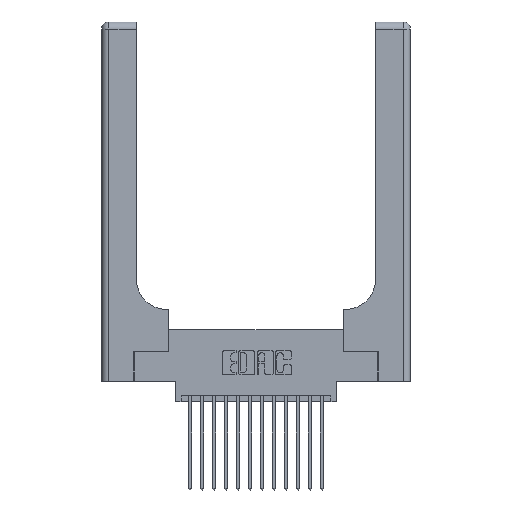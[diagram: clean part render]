
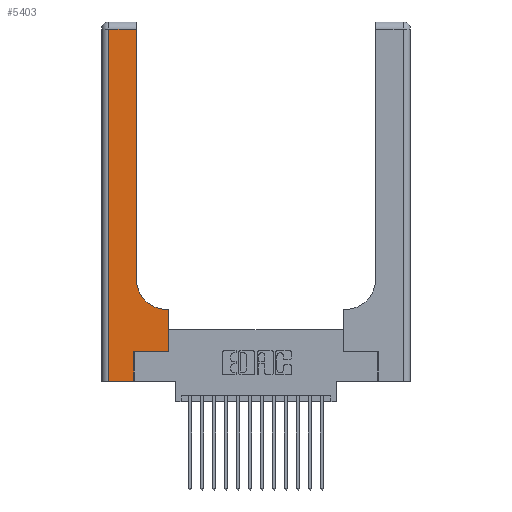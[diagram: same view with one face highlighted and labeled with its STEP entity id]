
A CAD part, top view. The second image highlights one B-rep face of the part: STEP entity #5403.
In plain terms, the highlighted planar face has unit normal (0, 0, 1).
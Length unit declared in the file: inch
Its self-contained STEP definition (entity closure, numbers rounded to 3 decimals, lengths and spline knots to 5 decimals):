
#266 = CARTESIAN_POINT ( 'NONE',  ( 0.269, 0.25, 0.37 ) ) ;
#598 = DIRECTION ( 'NONE',  ( -1., 0., 0. ) ) ;
#629 = CARTESIAN_POINT ( 'NONE',  ( 0.5585, 0.6, 0.37 ) ) ;
#652 = VECTOR ( 'NONE', #2944, 39.37008 ) ;
#919 = EDGE_CURVE ( 'NONE', #15310, #13263, #16381, .T. ) ;
#1130 = DIRECTION ( 'NONE',  ( 0., 1., 0. ) ) ;
#1141 = LINE ( 'NONE', #266, #12323 ) ;
#1341 = ORIENTED_EDGE ( 'NONE', *, *, #3066, .T. ) ;
#1475 = ORIENTED_EDGE ( 'NONE', *, *, #15976, .T. ) ;
#1748 = DIRECTION ( 'NONE',  ( 1., 0., 0. ) ) ;
#1870 = VERTEX_POINT ( 'NONE', #4251 ) ;
#1948 = LINE ( 'NONE', #5599, #9710 ) ;
#2033 = LINE ( 'NONE', #13127, #652 ) ;
#2573 = CIRCLE ( 'NONE', #14750, 0.25 ) ;
#2944 = DIRECTION ( 'NONE',  ( 0., 1., 0. ) ) ;
#3066 = EDGE_CURVE ( 'NONE', #6916, #9124, #1948, .T. ) ;
#3517 = PLANE ( 'NONE',  #14781 ) ;
#3930 = DIRECTION ( 'NONE',  ( -1., 0., 0. ) ) ;
#4251 = CARTESIAN_POINT ( 'NONE',  ( 0.2915, 2.94, 0.37 ) ) ;
#4790 = CARTESIAN_POINT ( 'NONE',  ( 0., 2.94, 0.37 ) ) ;
#4923 = ORIENTED_EDGE ( 'NONE', *, *, #16850, .T. ) ;
#5403 = ADVANCED_FACE ( 'NONE', ( #16533 ), #3517, .F. ) ;
#5599 = CARTESIAN_POINT ( 'NONE',  ( 0.269, 0., 0.37 ) ) ;
#5705 = ORIENTED_EDGE ( 'NONE', *, *, #14461, .T. ) ;
#6090 = CARTESIAN_POINT ( 'NONE',  ( 0.06, 2.94, 0.37 ) ) ;
#6234 = DIRECTION ( 'NONE',  ( -1., 0., 0. ) ) ;
#6240 = ORIENTED_EDGE ( 'NONE', *, *, #919, .T. ) ;
#6687 = CARTESIAN_POINT ( 'NONE',  ( 0.269, 0.25, 0.37 ) ) ;
#6916 = VERTEX_POINT ( 'NONE', #15922 ) ;
#7087 = EDGE_LOOP ( 'NONE', ( #4923, #15583, #6240, #9224, #1341, #1475, #16761, #13701, #5705 ) ) ;
#7119 = CARTESIAN_POINT ( 'NONE',  ( 0.06, 0., 0.37 ) ) ;
#7255 = CARTESIAN_POINT ( 'NONE',  ( 0.5415, 0.85, 0.37 ) ) ;
#7852 = EDGE_CURVE ( 'NONE', #13263, #6916, #12574, .T. ) ;
#8711 = DIRECTION ( 'NONE',  ( 1., 0., 0. ) ) ;
#8785 = LINE ( 'NONE', #12603, #12173 ) ;
#8894 = VECTOR ( 'NONE', #12679, 39.37008 ) ;
#9124 = VERTEX_POINT ( 'NONE', #6687 ) ;
#9224 = ORIENTED_EDGE ( 'NONE', *, *, #7852, .T. ) ;
#9353 = DIRECTION ( 'NONE',  ( 0., 0., -1. ) ) ;
#9564 = VECTOR ( 'NONE', #6234, 39.37008 ) ;
#9710 = VECTOR ( 'NONE', #1130, 39.37008 ) ;
#10383 = CARTESIAN_POINT ( 'NONE',  ( 0.5585, 0.25, 0.37 ) ) ;
#10666 = CARTESIAN_POINT ( 'NONE',  ( 0., 3., 0.37 ) ) ;
#10747 = VERTEX_POINT ( 'NONE', #16953 ) ;
#11168 = DIRECTION ( 'NONE',  ( 0., -1., 0. ) ) ;
#11378 = CARTESIAN_POINT ( 'NONE',  ( 0.06, 3., 0.37 ) ) ;
#12164 = VERTEX_POINT ( 'NONE', #17160 ) ;
#12173 = VECTOR ( 'NONE', #3930, 39.37008 ) ;
#12323 = VECTOR ( 'NONE', #1748, 39.37008 ) ;
#12574 = LINE ( 'NONE', #15379, #15992 ) ;
#12603 = CARTESIAN_POINT ( 'NONE',  ( 0.2915, 0.6, 0.37 ) ) ;
#12679 = DIRECTION ( 'NONE',  ( 0., 1., 0. ) ) ;
#12742 = LINE ( 'NONE', #16988, #8894 ) ;
#12966 = VECTOR ( 'NONE', #11168, 39.37008 ) ;
#13127 = CARTESIAN_POINT ( 'NONE',  ( 0.5585, 0.25, 0.37 ) ) ;
#13263 = VERTEX_POINT ( 'NONE', #7119 ) ;
#13701 = ORIENTED_EDGE ( 'NONE', *, *, #13795, .T. ) ;
#13795 = EDGE_CURVE ( 'NONE', #16691, #10747, #8785, .T. ) ;
#14461 = EDGE_CURVE ( 'NONE', #10747, #12164, #2573, .T. ) ;
#14637 = VERTEX_POINT ( 'NONE', #10383 ) ;
#14750 = AXIS2_PLACEMENT_3D ( 'NONE', #7255, #17382, #8711 ) ;
#14781 = AXIS2_PLACEMENT_3D ( 'NONE', #10666, #9353, #598 ) ;
#15310 = VERTEX_POINT ( 'NONE', #6090 ) ;
#15379 = CARTESIAN_POINT ( 'NONE',  ( 0., 0., 0.37 ) ) ;
#15583 = ORIENTED_EDGE ( 'NONE', *, *, #17746, .T. ) ;
#15922 = CARTESIAN_POINT ( 'NONE',  ( 0.269, 0., 0.37 ) ) ;
#15976 = EDGE_CURVE ( 'NONE', #9124, #14637, #1141, .T. ) ;
#15992 = VECTOR ( 'NONE', #18198, 39.37008 ) ;
#16381 = LINE ( 'NONE', #11378, #12966 ) ;
#16533 = FACE_OUTER_BOUND ( 'NONE', #7087, .T. ) ;
#16691 = VERTEX_POINT ( 'NONE', #629 ) ;
#16761 = ORIENTED_EDGE ( 'NONE', *, *, #17608, .T. ) ;
#16850 = EDGE_CURVE ( 'NONE', #12164, #1870, #12742, .T. ) ;
#16953 = CARTESIAN_POINT ( 'NONE',  ( 0.5415, 0.6, 0.37 ) ) ;
#16988 = CARTESIAN_POINT ( 'NONE',  ( 0.2915, 3., 0.37 ) ) ;
#17160 = CARTESIAN_POINT ( 'NONE',  ( 0.2915, 0.85, 0.37 ) ) ;
#17272 = LINE ( 'NONE', #4790, #9564 ) ;
#17382 = DIRECTION ( 'NONE',  ( 0., 0., -1. ) ) ;
#17608 = EDGE_CURVE ( 'NONE', #14637, #16691, #2033, .T. ) ;
#17746 = EDGE_CURVE ( 'NONE', #1870, #15310, #17272, .T. ) ;
#18198 = DIRECTION ( 'NONE',  ( 1., 0., 0. ) ) ;
